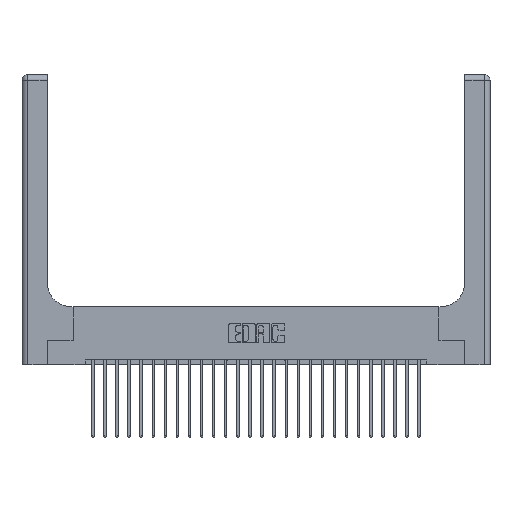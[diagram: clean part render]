
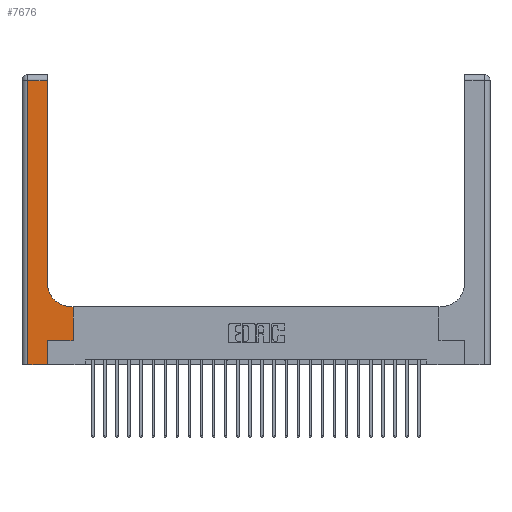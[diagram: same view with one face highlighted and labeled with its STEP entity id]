
A CAD part, top view. The second image highlights one B-rep face of the part: STEP entity #7676.
In plain terms, the highlighted planar face has unit normal (0, 0, 1).
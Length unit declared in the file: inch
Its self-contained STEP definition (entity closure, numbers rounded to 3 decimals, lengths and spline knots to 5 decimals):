
#373 = LINE ( 'NONE', #8324, #8193 ) ;
#1543 = CARTESIAN_POINT ( 'NONE',  ( 0.265, 0., 0.37 ) ) ;
#1923 = VERTEX_POINT ( 'NONE', #1543 ) ;
#2095 = ORIENTED_EDGE ( 'NONE', *, *, #6942, .T. ) ;
#2398 = EDGE_CURVE ( 'NONE', #18656, #21987, #3796, .T. ) ;
#2819 = DIRECTION ( 'NONE',  ( 0., 0., -1. ) ) ;
#2875 = DIRECTION ( 'NONE',  ( 1., 0., 0. ) ) ;
#2978 = LINE ( 'NONE', #18668, #20611 ) ;
#3132 = CARTESIAN_POINT ( 'NONE',  ( 0., 2.94, 0.37 ) ) ;
#3232 = DIRECTION ( 'NONE',  ( 0., 1., 0. ) ) ;
#3320 = ORIENTED_EDGE ( 'NONE', *, *, #22684, .T. ) ;
#3796 = LINE ( 'NONE', #17259, #12421 ) ;
#3875 = ORIENTED_EDGE ( 'NONE', *, *, #14780, .T. ) ;
#4573 = ORIENTED_EDGE ( 'NONE', *, *, #13812, .T. ) ;
#4786 = CARTESIAN_POINT ( 'NONE',  ( 0.51, 0.85, 0.37 ) ) ;
#4867 = DIRECTION ( 'NONE',  ( -1., 0., 0. ) ) ;
#4996 = CARTESIAN_POINT ( 'NONE',  ( 0.26, 0.6, 0.37 ) ) ;
#5660 = VERTEX_POINT ( 'NONE', #6764 ) ;
#5857 = CARTESIAN_POINT ( 'NONE',  ( 0.26, 2.94, 0.37 ) ) ;
#5871 = VERTEX_POINT ( 'NONE', #15906 ) ;
#6764 = CARTESIAN_POINT ( 'NONE',  ( 0.51, 0.6, 0.37 ) ) ;
#6865 = AXIS2_PLACEMENT_3D ( 'NONE', #4786, #2819, #16683 ) ;
#6942 = EDGE_CURVE ( 'NONE', #21987, #13312, #25097, .T. ) ;
#6963 = CARTESIAN_POINT ( 'NONE',  ( 0.26, 0.85, 0.37 ) ) ;
#7676 = ADVANCED_FACE ( 'NONE', ( #22149 ), #12236, .F. ) ;
#7779 = EDGE_CURVE ( 'NONE', #5660, #18656, #18130, .T. ) ;
#8193 = VECTOR ( 'NONE', #12510, 39.37008 ) ;
#8314 = DIRECTION ( 'NONE',  ( 0., 0., -1. ) ) ;
#8324 = CARTESIAN_POINT ( 'NONE',  ( 0.265, 0., 0.37 ) ) ;
#8387 = DIRECTION ( 'NONE',  ( 0., -1., 0. ) ) ;
#8546 = ORIENTED_EDGE ( 'NONE', *, *, #20678, .T. ) ;
#8916 = ORIENTED_EDGE ( 'NONE', *, *, #2398, .T. ) ;
#9646 = CARTESIAN_POINT ( 'NONE',  ( 0.06, 2.94, 0.37 ) ) ;
#10594 = ORIENTED_EDGE ( 'NONE', *, *, #7779, .T. ) ;
#11335 = EDGE_CURVE ( 'NONE', #13312, #5871, #12704, .T. ) ;
#11349 = VECTOR ( 'NONE', #24966, 39.37008 ) ;
#11358 = DIRECTION ( 'NONE',  ( -1., 0., 0. ) ) ;
#12089 = CARTESIAN_POINT ( 'NONE',  ( 0.265, 0.25, 0.37 ) ) ;
#12236 = PLANE ( 'NONE',  #25223 ) ;
#12421 = VECTOR ( 'NONE', #13468, 39.37008 ) ;
#12510 = DIRECTION ( 'NONE',  ( 0., 1., 0. ) ) ;
#12704 = LINE ( 'NONE', #14536, #24418 ) ;
#12972 = VERTEX_POINT ( 'NONE', #18290 ) ;
#13312 = VERTEX_POINT ( 'NONE', #9646 ) ;
#13468 = DIRECTION ( 'NONE',  ( 0., 1., 0. ) ) ;
#13812 = EDGE_CURVE ( 'NONE', #19938, #5660, #24855, .T. ) ;
#13855 = ORIENTED_EDGE ( 'NONE', *, *, #17633, .T. ) ;
#14189 = DIRECTION ( 'NONE',  ( 1., 0., 0. ) ) ;
#14536 = CARTESIAN_POINT ( 'NONE',  ( 0.06, 3., 0.37 ) ) ;
#14754 = ORIENTED_EDGE ( 'NONE', *, *, #11335, .T. ) ;
#14780 = EDGE_CURVE ( 'NONE', #5871, #1923, #14920, .T. ) ;
#14920 = LINE ( 'NONE', #16608, #15758 ) ;
#14938 = VERTEX_POINT ( 'NONE', #18625 ) ;
#15758 = VECTOR ( 'NONE', #2875, 39.37008 ) ;
#15906 = CARTESIAN_POINT ( 'NONE',  ( 0.06, 0., 0.37 ) ) ;
#16147 = LINE ( 'NONE', #12089, #25675 ) ;
#16608 = CARTESIAN_POINT ( 'NONE',  ( 0., 0., 0.37 ) ) ;
#16683 = DIRECTION ( 'NONE',  ( 1., 0., 0. ) ) ;
#17259 = CARTESIAN_POINT ( 'NONE',  ( 0.26, 3., 0.37 ) ) ;
#17633 = EDGE_CURVE ( 'NONE', #12972, #19938, #2978, .T. ) ;
#17862 = CARTESIAN_POINT ( 'NONE',  ( 0., 3., 0.37 ) ) ;
#18130 = CIRCLE ( 'NONE', #6865, 0.25 ) ;
#18290 = CARTESIAN_POINT ( 'NONE',  ( 0.528, 0.25, 0.37 ) ) ;
#18625 = CARTESIAN_POINT ( 'NONE',  ( 0.265, 0.25, 0.37 ) ) ;
#18656 = VERTEX_POINT ( 'NONE', #6963 ) ;
#18668 = CARTESIAN_POINT ( 'NONE',  ( 0.528, 0.25, 0.37 ) ) ;
#19624 = CARTESIAN_POINT ( 'NONE',  ( 0.528, 0.6, 0.37 ) ) ;
#19938 = VERTEX_POINT ( 'NONE', #19624 ) ;
#20611 = VECTOR ( 'NONE', #3232, 39.37008 ) ;
#20678 = EDGE_CURVE ( 'NONE', #14938, #12972, #16147, .T. ) ;
#21060 = EDGE_LOOP ( 'NONE', ( #8916, #2095, #14754, #3875, #3320, #8546, #13855, #4573, #10594 ) ) ;
#21596 = VECTOR ( 'NONE', #4867, 39.37008 ) ;
#21987 = VERTEX_POINT ( 'NONE', #5857 ) ;
#22149 = FACE_OUTER_BOUND ( 'NONE', #21060, .T. ) ;
#22684 = EDGE_CURVE ( 'NONE', #1923, #14938, #373, .T. ) ;
#24418 = VECTOR ( 'NONE', #8387, 39.37008 ) ;
#24855 = LINE ( 'NONE', #4996, #21596 ) ;
#24966 = DIRECTION ( 'NONE',  ( -1., 0., 0. ) ) ;
#25097 = LINE ( 'NONE', #3132, #11349 ) ;
#25223 = AXIS2_PLACEMENT_3D ( 'NONE', #17862, #8314, #11358 ) ;
#25675 = VECTOR ( 'NONE', #14189, 39.37008 ) ;
